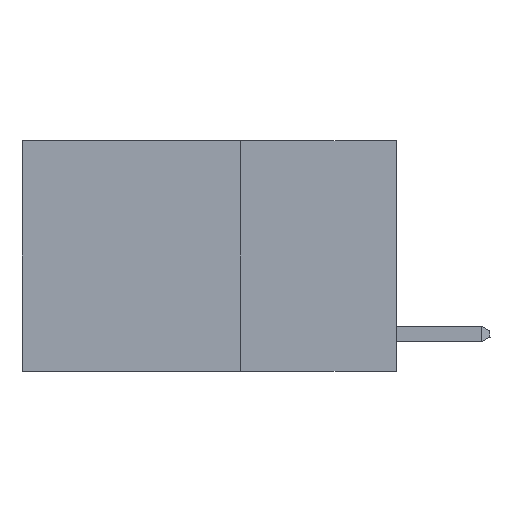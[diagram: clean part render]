
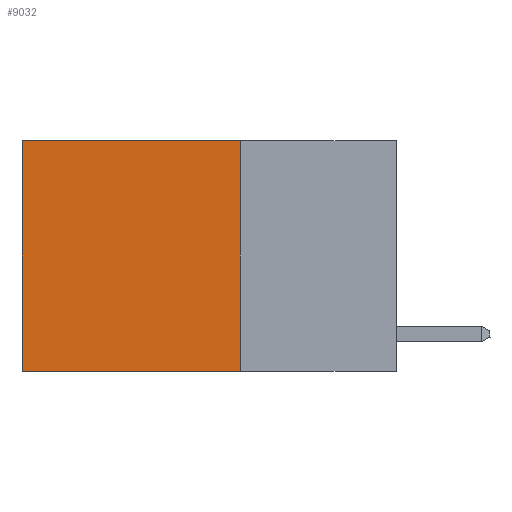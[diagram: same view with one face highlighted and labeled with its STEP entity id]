
A CAD part, left-side view. The second image highlights one B-rep face of the part: STEP entity #9032.
In plain terms, the highlighted planar face has unit normal (-1, 0, 0).
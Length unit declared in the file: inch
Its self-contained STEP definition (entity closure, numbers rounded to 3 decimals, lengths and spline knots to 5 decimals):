
#79 = VECTOR ( 'NONE', #930, 39.37008 ) ;
#306 = VERTEX_POINT ( 'NONE', #7839 ) ;
#383 = CARTESIAN_POINT ( 'NONE',  ( 0.2625, 0.25, 0. ) ) ;
#473 = ORIENTED_EDGE ( 'NONE', *, *, #9500, .F. ) ;
#930 = DIRECTION ( 'NONE',  ( 0., 0., -1. ) ) ;
#956 = VERTEX_POINT ( 'NONE', #1071 ) ;
#1071 = CARTESIAN_POINT ( 'NONE',  ( 0.2625, 0.25, 0. ) ) ;
#1182 = DIRECTION ( 'NONE',  ( 0., 1., 0. ) ) ;
#2007 = CARTESIAN_POINT ( 'NONE',  ( 0.2625, 0.6, 0. ) ) ;
#2069 = CARTESIAN_POINT ( 'NONE',  ( 0.2625, 0.25, -0.37 ) ) ;
#2592 = ORIENTED_EDGE ( 'NONE', *, *, #7467, .T. ) ;
#2845 = VECTOR ( 'NONE', #9999, 39.37008 ) ;
#3700 = CARTESIAN_POINT ( 'NONE',  ( 0.2625, 0.25, 0. ) ) ;
#3901 = VECTOR ( 'NONE', #1182, 39.37008 ) ;
#3966 = VERTEX_POINT ( 'NONE', #10054 ) ;
#4324 = EDGE_LOOP ( 'NONE', ( #2592, #473, #9226, #7735 ) ) ;
#4947 = LINE ( 'NONE', #6610, #8881 ) ;
#5097 = CARTESIAN_POINT ( 'NONE',  ( 0.2625, 0.25, -0.37 ) ) ;
#5208 = DIRECTION ( 'NONE',  ( 1., 0., 0. ) ) ;
#5653 = EDGE_CURVE ( 'NONE', #956, #8820, #7674, .T. ) ;
#5864 = LINE ( 'NONE', #2007, #79 ) ;
#5890 = LINE ( 'NONE', #5097, #3901 ) ;
#6127 = EDGE_CURVE ( 'NONE', #956, #306, #4947, .T. ) ;
#6610 = CARTESIAN_POINT ( 'NONE',  ( 0.2625, 0.25, 0. ) ) ;
#6617 = AXIS2_PLACEMENT_3D ( 'NONE', #3700, #5208, #7599 ) ;
#7467 = EDGE_CURVE ( 'NONE', #306, #3966, #5864, .T. ) ;
#7599 = DIRECTION ( 'NONE',  ( 0., 0., -1. ) ) ;
#7674 = LINE ( 'NONE', #383, #2845 ) ;
#7735 = ORIENTED_EDGE ( 'NONE', *, *, #6127, .T. ) ;
#7749 = FACE_OUTER_BOUND ( 'NONE', #4324, .T. ) ;
#7839 = CARTESIAN_POINT ( 'NONE',  ( 0.2625, 0.6, 0. ) ) ;
#8820 = VERTEX_POINT ( 'NONE', #2069 ) ;
#8881 = VECTOR ( 'NONE', #8887, 39.37008 ) ;
#8887 = DIRECTION ( 'NONE',  ( 0., 1., 0. ) ) ;
#9032 = ADVANCED_FACE ( 'NONE', ( #7749 ), #9323, .F. ) ;
#9226 = ORIENTED_EDGE ( 'NONE', *, *, #5653, .F. ) ;
#9323 = PLANE ( 'NONE',  #6617 ) ;
#9500 = EDGE_CURVE ( 'NONE', #8820, #3966, #5890, .T. ) ;
#9999 = DIRECTION ( 'NONE',  ( 0., 0., -1. ) ) ;
#10054 = CARTESIAN_POINT ( 'NONE',  ( 0.2625, 0.6, -0.37 ) ) ;
